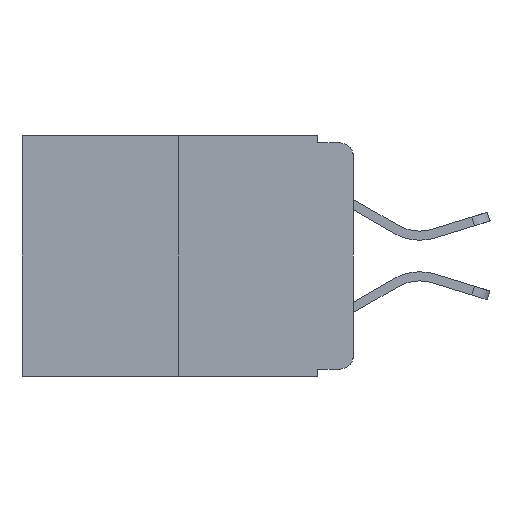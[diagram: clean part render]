
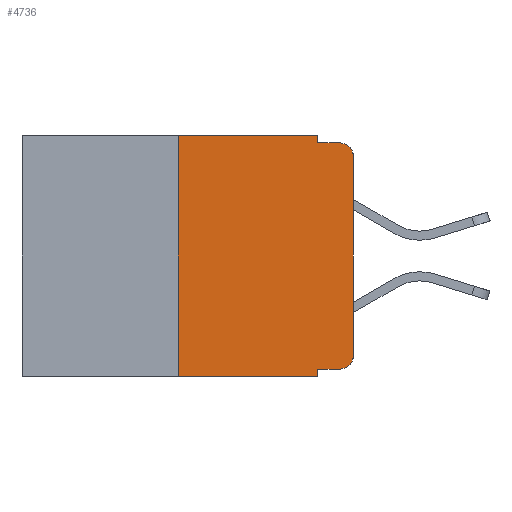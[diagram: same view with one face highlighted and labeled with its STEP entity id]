
A CAD part, left-side view. The second image highlights one B-rep face of the part: STEP entity #4736.
In plain terms, the highlighted planar face has unit normal (-1, 0, 0).
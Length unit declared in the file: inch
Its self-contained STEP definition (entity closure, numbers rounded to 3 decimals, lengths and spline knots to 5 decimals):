
#218 = LINE ( 'NONE', #10240, #9823 ) ;
#241 = CARTESIAN_POINT ( 'NONE',  ( 0., 0.02, -0.01 ) ) ;
#260 = CARTESIAN_POINT ( 'NONE',  ( 0., 0.051, -0.343 ) ) ;
#438 = EDGE_CURVE ( 'NONE', #2079, #10663, #8633, .T. ) ;
#525 = VERTEX_POINT ( 'NONE', #241 ) ;
#675 = AXIS2_PLACEMENT_3D ( 'NONE', #6121, #4371, #4326 ) ;
#986 = EDGE_CURVE ( 'NONE', #10201, #9761, #218, .T. ) ;
#1128 = CARTESIAN_POINT ( 'NONE',  ( 0., 0.051, -0.01 ) ) ;
#1202 = LINE ( 'NONE', #4111, #10591 ) ;
#1378 = CARTESIAN_POINT ( 'NONE',  ( 0., 0.051, 0. ) ) ;
#1384 = ORIENTED_EDGE ( 'NONE', *, *, #3429, .F. ) ;
#1416 = DIRECTION ( 'NONE',  ( 0., 0., -1. ) ) ;
#1458 = ORIENTED_EDGE ( 'NONE', *, *, #2775, .T. ) ;
#1487 = EDGE_CURVE ( 'NONE', #9761, #2662, #8766, .T. ) ;
#1515 = ORIENTED_EDGE ( 'NONE', *, *, #1487, .F. ) ;
#1589 = ORIENTED_EDGE ( 'NONE', *, *, #1657, .T. ) ;
#1618 = EDGE_CURVE ( 'NONE', #2662, #525, #1202, .T. ) ;
#1637 = EDGE_CURVE ( 'NONE', #10663, #525, #8329, .T. ) ;
#1646 = VERTEX_POINT ( 'NONE', #2446 ) ;
#1657 = EDGE_CURVE ( 'NONE', #3549, #1908, #3342, .T. ) ;
#1908 = VERTEX_POINT ( 'NONE', #10400 ) ;
#1931 = ORIENTED_EDGE ( 'NONE', *, *, #1637, .T. ) ;
#1937 = FACE_OUTER_BOUND ( 'NONE', #2260, .T. ) ;
#1986 = VECTOR ( 'NONE', #2046, 39.37008 ) ;
#2046 = DIRECTION ( 'NONE',  ( 0., -1., 0. ) ) ;
#2079 = VERTEX_POINT ( 'NONE', #3535 ) ;
#2260 = EDGE_LOOP ( 'NONE', ( #4807, #1931, #9194, #1515, #3252, #2265, #1458, #1384, #1589, #3562 ) ) ;
#2265 = ORIENTED_EDGE ( 'NONE', *, *, #3350, .F. ) ;
#2446 = CARTESIAN_POINT ( 'NONE',  ( 0., 0.25, -0.343 ) ) ;
#2481 = DIRECTION ( 'NONE',  ( 0., -1., 0. ) ) ;
#2662 = VERTEX_POINT ( 'NONE', #1128 ) ;
#2775 = EDGE_CURVE ( 'NONE', #1646, #6441, #6914, .T. ) ;
#3252 = ORIENTED_EDGE ( 'NONE', *, *, #986, .F. ) ;
#3309 = EDGE_CURVE ( 'NONE', #1908, #2079, #6310, .T. ) ;
#3342 = LINE ( 'NONE', #8804, #10319 ) ;
#3350 = EDGE_CURVE ( 'NONE', #1646, #10201, #6032, .T. ) ;
#3429 = EDGE_CURVE ( 'NONE', #3549, #6441, #7297, .T. ) ;
#3516 = CARTESIAN_POINT ( 'NONE',  ( 0., 0.02, -0.313 ) ) ;
#3535 = CARTESIAN_POINT ( 'NONE',  ( 0., 0., -0.313 ) ) ;
#3549 = VERTEX_POINT ( 'NONE', #9912 ) ;
#3562 = ORIENTED_EDGE ( 'NONE', *, *, #3309, .T. ) ;
#3771 = DIRECTION ( 'NONE',  ( 0., 0., -1. ) ) ;
#3881 = CARTESIAN_POINT ( 'NONE',  ( 0., 0.25, 0. ) ) ;
#3996 = DIRECTION ( 'NONE',  ( -1., 0., 0. ) ) ;
#4111 = CARTESIAN_POINT ( 'NONE',  ( 0., 0.051, -0.01 ) ) ;
#4326 = DIRECTION ( 'NONE',  ( 0., 0., -1. ) ) ;
#4371 = DIRECTION ( 'NONE',  ( 1., 0., 0. ) ) ;
#4736 = ADVANCED_FACE ( 'NONE', ( #1937 ), #9820, .F. ) ;
#4807 = ORIENTED_EDGE ( 'NONE', *, *, #438, .T. ) ;
#4908 = DIRECTION ( 'NONE',  ( 0., 0., 1. ) ) ;
#5640 = CARTESIAN_POINT ( 'NONE',  ( 0., 0.051, 0. ) ) ;
#5664 = DIRECTION ( 'NONE',  ( 0., 0., -1. ) ) ;
#5938 = DIRECTION ( 'NONE',  ( 0., 0., 1. ) ) ;
#5982 = VECTOR ( 'NONE', #4908, 39.37008 ) ;
#6032 = LINE ( 'NONE', #11210, #10391 ) ;
#6104 = CARTESIAN_POINT ( 'NONE',  ( 0., 0., -0.03 ) ) ;
#6121 = CARTESIAN_POINT ( 'NONE',  ( 0., 0.473, 0. ) ) ;
#6310 = CIRCLE ( 'NONE', #11688, 0.02 ) ;
#6441 = VERTEX_POINT ( 'NONE', #260 ) ;
#6602 = DIRECTION ( 'NONE',  ( 0., 0., -1. ) ) ;
#6701 = DIRECTION ( 'NONE',  ( 0., -1., 0. ) ) ;
#6731 = AXIS2_PLACEMENT_3D ( 'NONE', #7078, #10737, #6602 ) ;
#6914 = LINE ( 'NONE', #11375, #1986 ) ;
#7078 = CARTESIAN_POINT ( 'NONE',  ( 0., 0.02, -0.03 ) ) ;
#7297 = LINE ( 'NONE', #5640, #11275 ) ;
#8194 = VECTOR ( 'NONE', #1416, 39.37008 ) ;
#8329 = CIRCLE ( 'NONE', #6731, 0.02 ) ;
#8633 = LINE ( 'NONE', #11395, #5982 ) ;
#8766 = LINE ( 'NONE', #1378, #8194 ) ;
#8804 = CARTESIAN_POINT ( 'NONE',  ( 0., 0.051, -0.333 ) ) ;
#9194 = ORIENTED_EDGE ( 'NONE', *, *, #1618, .F. ) ;
#9470 = CARTESIAN_POINT ( 'NONE',  ( 0., 0.051, 0. ) ) ;
#9761 = VERTEX_POINT ( 'NONE', #9470 ) ;
#9820 = PLANE ( 'NONE',  #675 ) ;
#9823 = VECTOR ( 'NONE', #10529, 39.37008 ) ;
#9912 = CARTESIAN_POINT ( 'NONE',  ( 0., 0.051, -0.333 ) ) ;
#10201 = VERTEX_POINT ( 'NONE', #3881 ) ;
#10240 = CARTESIAN_POINT ( 'NONE',  ( 0., 0.473, 0. ) ) ;
#10319 = VECTOR ( 'NONE', #2481, 39.37008 ) ;
#10391 = VECTOR ( 'NONE', #5938, 39.37008 ) ;
#10400 = CARTESIAN_POINT ( 'NONE',  ( 0., 0.02, -0.333 ) ) ;
#10529 = DIRECTION ( 'NONE',  ( 0., -1., 0. ) ) ;
#10591 = VECTOR ( 'NONE', #6701, 39.37008 ) ;
#10663 = VERTEX_POINT ( 'NONE', #6104 ) ;
#10737 = DIRECTION ( 'NONE',  ( -1., 0., 0. ) ) ;
#11210 = CARTESIAN_POINT ( 'NONE',  ( 0., 0.25, 0. ) ) ;
#11275 = VECTOR ( 'NONE', #5664, 39.37008 ) ;
#11375 = CARTESIAN_POINT ( 'NONE',  ( 0., 0.473, -0.343 ) ) ;
#11395 = CARTESIAN_POINT ( 'NONE',  ( 0., 0., 0. ) ) ;
#11688 = AXIS2_PLACEMENT_3D ( 'NONE', #3516, #3996, #3771 ) ;
